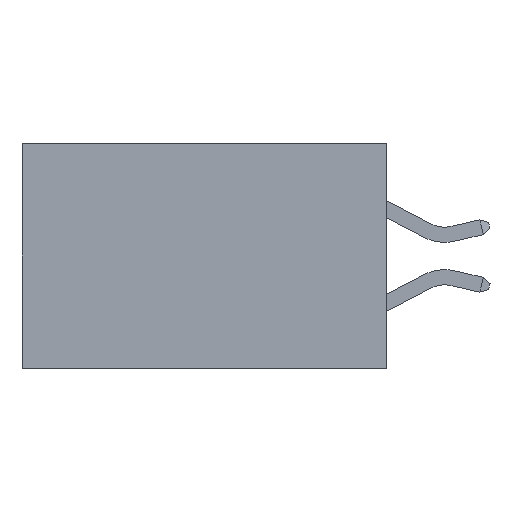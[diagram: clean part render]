
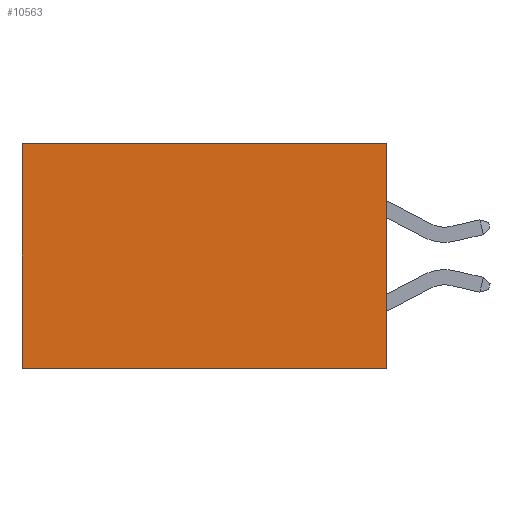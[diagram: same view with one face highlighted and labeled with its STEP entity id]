
A CAD part, left-side view. The second image highlights one B-rep face of the part: STEP entity #10563.
In plain terms, the highlighted planar face has unit normal (-1, 0, 0).
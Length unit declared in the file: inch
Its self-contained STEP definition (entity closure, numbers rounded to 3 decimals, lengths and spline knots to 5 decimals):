
#1158 = EDGE_CURVE ( 'NONE', #7812, #9635, #15794, .T. ) ;
#3109 = CARTESIAN_POINT ( 'NONE',  ( 0.298, 0., 0. ) ) ;
#3344 = VECTOR ( 'NONE', #8967, 39.37008 ) ;
#4012 = EDGE_LOOP ( 'NONE', ( #18711, #4450, #14942, #8920 ) ) ;
#4238 = EDGE_CURVE ( 'NONE', #7812, #8505, #12666, .T. ) ;
#4450 = ORIENTED_EDGE ( 'NONE', *, *, #7391, .F. ) ;
#4622 = CARTESIAN_POINT ( 'NONE',  ( 0.298, 0., -0.37 ) ) ;
#5157 = DIRECTION ( 'NONE',  ( 0., 0., -1. ) ) ;
#5387 = VECTOR ( 'NONE', #10366, 39.37008 ) ;
#6117 = VERTEX_POINT ( 'NONE', #12882 ) ;
#6391 = CARTESIAN_POINT ( 'NONE',  ( 0.298, 0., 0. ) ) ;
#7121 = CARTESIAN_POINT ( 'NONE',  ( 0.298, 0.6, 0. ) ) ;
#7391 = EDGE_CURVE ( 'NONE', #8505, #6117, #19074, .T. ) ;
#7455 = VECTOR ( 'NONE', #11795, 39.37008 ) ;
#7812 = VERTEX_POINT ( 'NONE', #13495 ) ;
#8089 = CARTESIAN_POINT ( 'NONE',  ( 0.298, 0., 0. ) ) ;
#8505 = VERTEX_POINT ( 'NONE', #20055 ) ;
#8657 = AXIS2_PLACEMENT_3D ( 'NONE', #8089, #13119, #5157 ) ;
#8920 = ORIENTED_EDGE ( 'NONE', *, *, #1158, .T. ) ;
#8967 = DIRECTION ( 'NONE',  ( 0., 0., -1. ) ) ;
#9544 = LINE ( 'NONE', #7121, #5387 ) ;
#9635 = VERTEX_POINT ( 'NONE', #20114 ) ;
#10366 = DIRECTION ( 'NONE',  ( 0., 0., -1. ) ) ;
#10563 = ADVANCED_FACE ( 'NONE', ( #11921 ), #12845, .F. ) ;
#11795 = DIRECTION ( 'NONE',  ( 0., 1., 0. ) ) ;
#11921 = FACE_OUTER_BOUND ( 'NONE', #4012, .T. ) ;
#12666 = LINE ( 'NONE', #3109, #3344 ) ;
#12845 = PLANE ( 'NONE',  #8657 ) ;
#12882 = CARTESIAN_POINT ( 'NONE',  ( 0.298, 0.6, -0.37 ) ) ;
#13119 = DIRECTION ( 'NONE',  ( 1., 0., 0. ) ) ;
#13495 = CARTESIAN_POINT ( 'NONE',  ( 0.298, 0., 0. ) ) ;
#13932 = VECTOR ( 'NONE', #20137, 39.37008 ) ;
#14942 = ORIENTED_EDGE ( 'NONE', *, *, #4238, .F. ) ;
#15794 = LINE ( 'NONE', #6391, #7455 ) ;
#18711 = ORIENTED_EDGE ( 'NONE', *, *, #19764, .T. ) ;
#19074 = LINE ( 'NONE', #4622, #13932 ) ;
#19764 = EDGE_CURVE ( 'NONE', #9635, #6117, #9544, .T. ) ;
#20055 = CARTESIAN_POINT ( 'NONE',  ( 0.298, 0., -0.37 ) ) ;
#20114 = CARTESIAN_POINT ( 'NONE',  ( 0.298, 0.6, 0. ) ) ;
#20137 = DIRECTION ( 'NONE',  ( 0., 1., 0. ) ) ;
